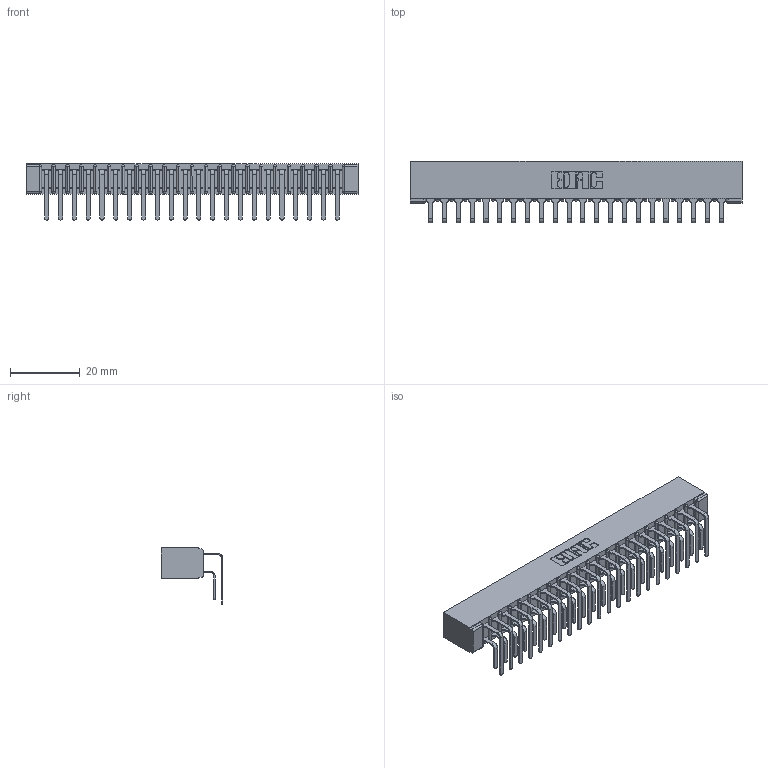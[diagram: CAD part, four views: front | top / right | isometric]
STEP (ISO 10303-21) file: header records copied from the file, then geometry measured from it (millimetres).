
FILE_DESCRIPTION (( 'STEP AP203' ), '1' );
FILE_NAME ('307-022-459-101.STEP', '2020-09-27T06:22:45', ( '' ), ( '' ), 'SwSTEP 2.0', 'SolidWorks 2020', '' );
FILE_SCHEMA (( 'CONFIG_CONTROL_DESIGN' ));
Length unit declared in the file: inch
Products named in the file (4): 307 Part_No Mounting Lugs; 307-290-001_559 - 2 (Single); 307-022-459-101; 307-290-001_558 559 - 1 (Single)
Assembly tree (45 placements, depth 2):
  307-022-459-101
    307 Part_No Mounting Lugs
    307-290-001_558 559 - 1 (Single)  x22
    307-290-001_559 - 2 (Single)  x22
Bounding box: 95.05 x 17.69 x 16.08 mm (x, y, z)
Volume: 6645.3 mm3; surface area: 13305.9 mm2
Topology: 45 solids, 45 shells, 2333 faces, 6547 edges, 4242 vertices
Faces by surface type: plane 1518, cylinder 769, sphere 46
Entity records: 23199 total; most frequent: CARTESIAN_POINT 3800, ORIENTED_EDGE 3762, DIRECTION 3729, EDGE_CURVE 1881, LINE 1435, VECTOR 1435, VERTEX_POINT 1218, AXIS2_PLACEMENT_3D 1147
